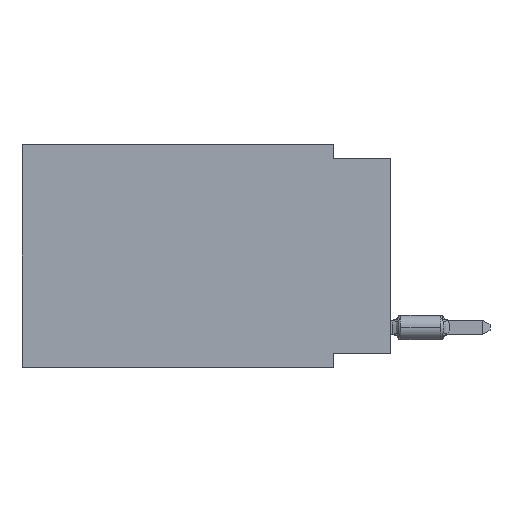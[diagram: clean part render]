
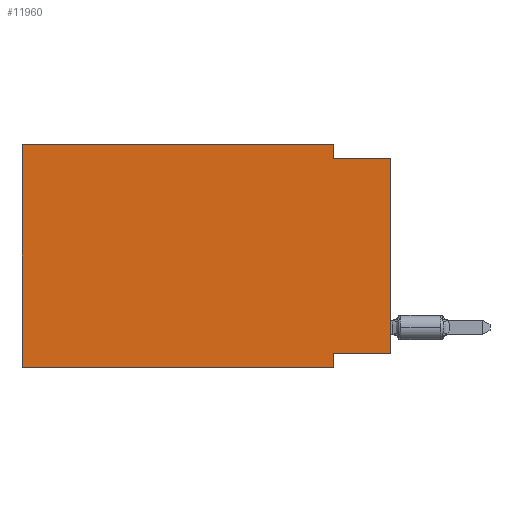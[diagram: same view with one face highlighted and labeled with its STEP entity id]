
A CAD part, left-side view. The second image highlights one B-rep face of the part: STEP entity #11960.
In plain terms, the highlighted planar face has unit normal (-1, 0, 0).
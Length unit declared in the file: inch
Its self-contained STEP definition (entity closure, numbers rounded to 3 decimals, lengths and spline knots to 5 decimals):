
#52 = VECTOR ( 'NONE', #19064, 39.37008 ) ;
#119 = LINE ( 'NONE', #17058, #7681 ) ;
#241 = CARTESIAN_POINT ( 'NONE',  ( 0., 0.645, 0. ) ) ;
#1231 = CARTESIAN_POINT ( 'NONE',  ( 0., 0., -0.025 ) ) ;
#1618 = VECTOR ( 'NONE', #6524, 39.37008 ) ;
#1869 = ORIENTED_EDGE ( 'NONE', *, *, #21214, .T. ) ;
#1893 = CARTESIAN_POINT ( 'NONE',  ( 0., 0.645, -0.39 ) ) ;
#2087 = CARTESIAN_POINT ( 'NONE',  ( 0., 0.1, -0.365 ) ) ;
#3328 = VECTOR ( 'NONE', #9192, 39.37008 ) ;
#3886 = CARTESIAN_POINT ( 'NONE',  ( 0., 0.1, 0. ) ) ;
#4041 = CARTESIAN_POINT ( 'NONE',  ( 0., 0.1, -0.025 ) ) ;
#5343 = DIRECTION ( 'NONE',  ( 0., 0., -1. ) ) ;
#5693 = FACE_OUTER_BOUND ( 'NONE', #8429, .T. ) ;
#5823 = EDGE_CURVE ( 'NONE', #26469, #11202, #14316, .T. ) ;
#6078 = VERTEX_POINT ( 'NONE', #2087 ) ;
#6460 = ORIENTED_EDGE ( 'NONE', *, *, #30683, .T. ) ;
#6524 = DIRECTION ( 'NONE',  ( 0., 0., 1. ) ) ;
#6828 = CARTESIAN_POINT ( 'NONE',  ( 0., 0.1, 0. ) ) ;
#7186 = LINE ( 'NONE', #35127, #52 ) ;
#7510 = VECTOR ( 'NONE', #15027, 39.37008 ) ;
#7681 = VECTOR ( 'NONE', #13615, 39.37008 ) ;
#8259 = CARTESIAN_POINT ( 'NONE',  ( 0., 0.1, -0.39 ) ) ;
#8429 = EDGE_LOOP ( 'NONE', ( #1869, #29074, #19413, #23005, #22320, #6460, #11165, #20832 ) ) ;
#8613 = DIRECTION ( 'NONE',  ( 1., 0., 0. ) ) ;
#9192 = DIRECTION ( 'NONE',  ( 0., -1., 0. ) ) ;
#9632 = CARTESIAN_POINT ( 'NONE',  ( 0., 0.645, -0.39 ) ) ;
#10319 = LINE ( 'NONE', #18740, #21899 ) ;
#11165 = ORIENTED_EDGE ( 'NONE', *, *, #25446, .F. ) ;
#11202 = VERTEX_POINT ( 'NONE', #1231 ) ;
#11695 = VERTEX_POINT ( 'NONE', #6828 ) ;
#11960 = ADVANCED_FACE ( 'NONE', ( #5693 ), #36030, .F. ) ;
#12096 = VERTEX_POINT ( 'NONE', #28303 ) ;
#12788 = EDGE_CURVE ( 'NONE', #31786, #6078, #119, .T. ) ;
#13615 = DIRECTION ( 'NONE',  ( 0., 1., 0. ) ) ;
#14316 = LINE ( 'NONE', #25419, #3328 ) ;
#15027 = DIRECTION ( 'NONE',  ( 0., 0., -1. ) ) ;
#16468 = LINE ( 'NONE', #8259, #24503 ) ;
#16796 = VERTEX_POINT ( 'NONE', #1893 ) ;
#17058 = CARTESIAN_POINT ( 'NONE',  ( 0., 0., -0.365 ) ) ;
#18136 = LINE ( 'NONE', #3886, #7510 ) ;
#18740 = CARTESIAN_POINT ( 'NONE',  ( 0., 0.645, 0. ) ) ;
#19052 = DIRECTION ( 'NONE',  ( 0., 0., -1. ) ) ;
#19064 = DIRECTION ( 'NONE',  ( 0., -1., 0. ) ) ;
#19413 = ORIENTED_EDGE ( 'NONE', *, *, #22969, .F. ) ;
#19692 = VERTEX_POINT ( 'NONE', #35054 ) ;
#20419 = DIRECTION ( 'NONE',  ( 0., 0., 1. ) ) ;
#20778 = DIRECTION ( 'NONE',  ( 0., -1., 0. ) ) ;
#20832 = ORIENTED_EDGE ( 'NONE', *, *, #12788, .F. ) ;
#21214 = EDGE_CURVE ( 'NONE', #31786, #11202, #31723, .T. ) ;
#21899 = VECTOR ( 'NONE', #20419, 39.37008 ) ;
#22320 = ORIENTED_EDGE ( 'NONE', *, *, #26797, .F. ) ;
#22969 = EDGE_CURVE ( 'NONE', #11695, #26469, #18136, .T. ) ;
#23005 = ORIENTED_EDGE ( 'NONE', *, *, #36027, .F. ) ;
#24503 = VECTOR ( 'NONE', #19052, 39.37008 ) ;
#25419 = CARTESIAN_POINT ( 'NONE',  ( 0., 0., -0.025 ) ) ;
#25446 = EDGE_CURVE ( 'NONE', #6078, #19692, #16468, .T. ) ;
#26229 = CARTESIAN_POINT ( 'NONE',  ( 0., 0., -0.365 ) ) ;
#26469 = VERTEX_POINT ( 'NONE', #4041 ) ;
#26797 = EDGE_CURVE ( 'NONE', #16796, #12096, #10319, .T. ) ;
#27825 = VECTOR ( 'NONE', #20778, 39.37008 ) ;
#28303 = CARTESIAN_POINT ( 'NONE',  ( 0., 0.645, 0. ) ) ;
#29074 = ORIENTED_EDGE ( 'NONE', *, *, #5823, .F. ) ;
#30683 = EDGE_CURVE ( 'NONE', #16796, #19692, #31352, .T. ) ;
#31352 = LINE ( 'NONE', #9632, #27825 ) ;
#31723 = LINE ( 'NONE', #34280, #1618 ) ;
#31786 = VERTEX_POINT ( 'NONE', #26229 ) ;
#33298 = AXIS2_PLACEMENT_3D ( 'NONE', #241, #8613, #5343 ) ;
#34280 = CARTESIAN_POINT ( 'NONE',  ( 0., 0., 0. ) ) ;
#35054 = CARTESIAN_POINT ( 'NONE',  ( 0., 0.1, -0.39 ) ) ;
#35127 = CARTESIAN_POINT ( 'NONE',  ( 0., 0.645, 0. ) ) ;
#36027 = EDGE_CURVE ( 'NONE', #12096, #11695, #7186, .T. ) ;
#36030 = PLANE ( 'NONE',  #33298 ) ;
